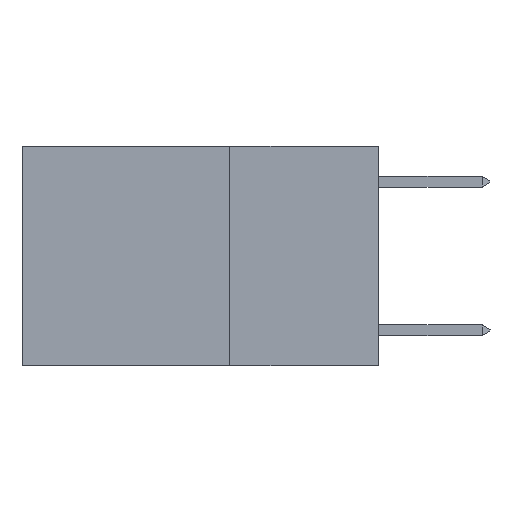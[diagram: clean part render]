
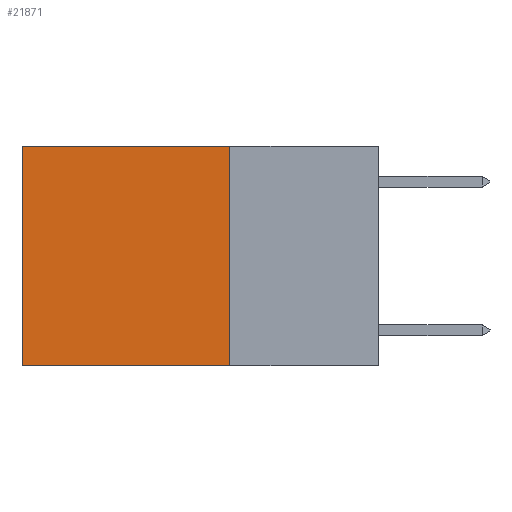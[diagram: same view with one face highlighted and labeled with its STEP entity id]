
A CAD part, left-side view. The second image highlights one B-rep face of the part: STEP entity #21871.
In plain terms, the highlighted planar face has unit normal (-1, 0, 0).
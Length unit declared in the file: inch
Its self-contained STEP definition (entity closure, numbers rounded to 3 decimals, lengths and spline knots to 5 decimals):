
#20 = CARTESIAN_POINT ( 'NONE',  ( 0.2625, 0.25, 0. ) ) ;
#1424 = DIRECTION ( 'NONE',  ( 0., 0., -1. ) ) ;
#1448 = DIRECTION ( 'NONE',  ( 1., 0., 0. ) ) ;
#1469 = CARTESIAN_POINT ( 'NONE',  ( 0.2625, 0.25, 0. ) ) ;
#1580 = PLANE ( 'NONE',  #3496 ) ;
#2369 = VECTOR ( 'NONE', #18812, 39.37008 ) ;
#2396 = LINE ( 'NONE', #19871, #2369 ) ;
#3496 = AXIS2_PLACEMENT_3D ( 'NONE', #1469, #1448, #1424 ) ;
#5184 = VERTEX_POINT ( 'NONE', #22015 ) ;
#5231 = EDGE_LOOP ( 'NONE', ( #17477, #21133, #13732, #8154 ) ) ;
#6085 = DIRECTION ( 'NONE',  ( 0., 1., 0. ) ) ;
#6370 = CARTESIAN_POINT ( 'NONE',  ( 0.2625, 0.25, 0. ) ) ;
#7310 = VECTOR ( 'NONE', #6085, 39.37008 ) ;
#8154 = ORIENTED_EDGE ( 'NONE', *, *, #20484, .T. ) ;
#8235 = VERTEX_POINT ( 'NONE', #21624 ) ;
#8854 = LINE ( 'NONE', #6370, #7310 ) ;
#12927 = CARTESIAN_POINT ( 'NONE',  ( 0.2625, 0.6, 0. ) ) ;
#13215 = DIRECTION ( 'NONE',  ( 0., 0., -1. ) ) ;
#13732 = ORIENTED_EDGE ( 'NONE', *, *, #21941, .F. ) ;
#14712 = LINE ( 'NONE', #20, #14857 ) ;
#14784 = EDGE_CURVE ( 'NONE', #5184, #15721, #2396, .T. ) ;
#14857 = VECTOR ( 'NONE', #23398, 39.37008 ) ;
#15365 = LINE ( 'NONE', #12927, #15455 ) ;
#15386 = FACE_OUTER_BOUND ( 'NONE', #5231, .T. ) ;
#15455 = VECTOR ( 'NONE', #13215, 39.37008 ) ;
#15721 = VERTEX_POINT ( 'NONE', #19087 ) ;
#15892 = EDGE_CURVE ( 'NONE', #16711, #15721, #15365, .T. ) ;
#16625 = CARTESIAN_POINT ( 'NONE',  ( 0.2625, 0.6, 0. ) ) ;
#16711 = VERTEX_POINT ( 'NONE', #16625 ) ;
#17477 = ORIENTED_EDGE ( 'NONE', *, *, #15892, .T. ) ;
#18812 = DIRECTION ( 'NONE',  ( 0., 1., 0. ) ) ;
#19087 = CARTESIAN_POINT ( 'NONE',  ( 0.2625, 0.6, -0.37 ) ) ;
#19871 = CARTESIAN_POINT ( 'NONE',  ( 0.2625, 0.25, -0.37 ) ) ;
#20484 = EDGE_CURVE ( 'NONE', #8235, #16711, #8854, .T. ) ;
#21133 = ORIENTED_EDGE ( 'NONE', *, *, #14784, .F. ) ;
#21624 = CARTESIAN_POINT ( 'NONE',  ( 0.2625, 0.25, 0. ) ) ;
#21871 = ADVANCED_FACE ( 'NONE', ( #15386 ), #1580, .F. ) ;
#21941 = EDGE_CURVE ( 'NONE', #8235, #5184, #14712, .T. ) ;
#22015 = CARTESIAN_POINT ( 'NONE',  ( 0.2625, 0.25, -0.37 ) ) ;
#23398 = DIRECTION ( 'NONE',  ( 0., 0., -1. ) ) ;
